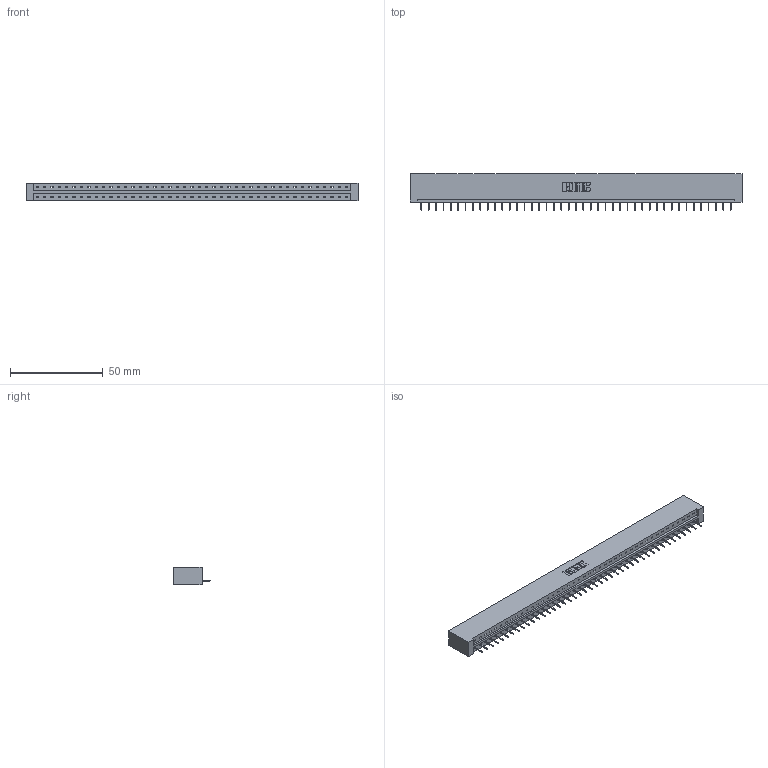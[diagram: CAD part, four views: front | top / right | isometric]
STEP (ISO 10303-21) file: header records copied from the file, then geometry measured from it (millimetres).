
FILE_DESCRIPTION (( 'STEP AP203' ), '1' );
FILE_NAME ('833-043-524-101.STEP', '2020-06-03T23:36:33', ( '' ), ( '' ), 'SwSTEP 2.0', 'SolidWorks 2020', '' );
FILE_SCHEMA (( 'CONFIG_CONTROL_DESIGN' ));
Length unit declared in the file: inch
Products named in the file (3): 833-043-524-101; 833 Part_Lugless; 345-292-001_345-293-124
Assembly tree (44 placements, depth 2):
  833-043-524-101
    833 Part_Lugless
    345-292-001_345-293-124  x43
Bounding box: 178.64 x 19.69 x 9.4 mm (x, y, z)
Volume: 18427.5 mm3; surface area: 19317.6 mm2
Topology: 44 solids, 44 shells, 2772 faces, 8027 edges, 5178 vertices
Faces by surface type: plane 2130, cylinder 642
Entity records: 25955 total; most frequent: CARTESIAN_POINT 4483, ORIENTED_EDGE 4462, DIRECTION 3773, EDGE_CURVE 2231, LINE 2115, VECTOR 2115, VERTEX_POINT 1482, AXIS2_PLACEMENT_3D 829
